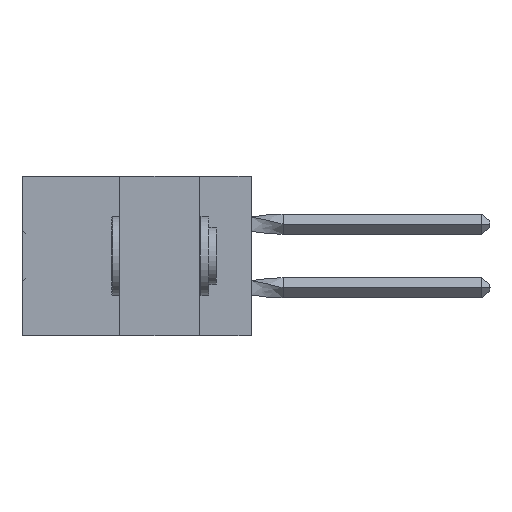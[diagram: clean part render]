
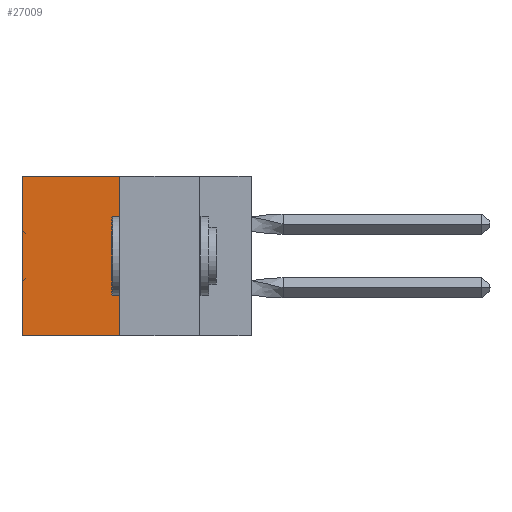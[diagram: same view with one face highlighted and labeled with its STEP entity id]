
A CAD part, left-side view. The second image highlights one B-rep face of the part: STEP entity #27009.
In plain terms, the highlighted planar face has unit normal (-1, 0, 0).
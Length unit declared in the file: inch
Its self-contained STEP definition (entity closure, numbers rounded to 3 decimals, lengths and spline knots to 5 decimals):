
#629 = VECTOR ( 'NONE', #10240, 39.37008 ) ;
#926 = ORIENTED_EDGE ( 'NONE', *, *, #4383, .F. ) ;
#1847 = CARTESIAN_POINT ( 'NONE',  ( 0.305, 0.413, -0.5 ) ) ;
#2015 = ORIENTED_EDGE ( 'NONE', *, *, #31952, .T. ) ;
#3936 = VERTEX_POINT ( 'NONE', #17953 ) ;
#4383 = EDGE_CURVE ( 'NONE', #3936, #9345, #38222, .T. ) ;
#5533 = EDGE_LOOP ( 'NONE', ( #58918, #926, #56568, #2015 ) ) ;
#8923 = VECTOR ( 'NONE', #50853, 39.37008 ) ;
#9345 = VERTEX_POINT ( 'NONE', #12733 ) ;
#10240 = DIRECTION ( 'NONE',  ( 0., 0., -1. ) ) ;
#10301 = LINE ( 'NONE', #25696, #34538 ) ;
#12241 = PLANE ( 'NONE',  #36626 ) ;
#12733 = CARTESIAN_POINT ( 'NONE',  ( 0.305, 0.72, -0.5 ) ) ;
#17953 = CARTESIAN_POINT ( 'NONE',  ( 0.305, 0.413, -0.5 ) ) ;
#19548 = CARTESIAN_POINT ( 'NONE',  ( 0.305, 0.413, -0.5 ) ) ;
#19824 = VERTEX_POINT ( 'NONE', #19971 ) ;
#19971 = CARTESIAN_POINT ( 'NONE',  ( 0.305, 0.413, 0. ) ) ;
#20335 = LINE ( 'NONE', #19548, #629 ) ;
#21225 = EDGE_CURVE ( 'NONE', #19824, #3936, #20335, .T. ) ;
#25521 = CARTESIAN_POINT ( 'NONE',  ( 0.305, 0.413, -0.5 ) ) ;
#25696 = CARTESIAN_POINT ( 'NONE',  ( 0.305, 0.72, -0.5 ) ) ;
#27009 = ADVANCED_FACE ( 'NONE', ( #57143 ), #12241, .F. ) ;
#31952 = EDGE_CURVE ( 'NONE', #19824, #47423, #58804, .T. ) ;
#34538 = VECTOR ( 'NONE', #59500, 39.37008 ) ;
#35964 = CARTESIAN_POINT ( 'NONE',  ( 0.305, 0.72, 0. ) ) ;
#36626 = AXIS2_PLACEMENT_3D ( 'NONE', #1847, #50872, #59964 ) ;
#36931 = CARTESIAN_POINT ( 'NONE',  ( 0.305, 0.413, 0. ) ) ;
#38222 = LINE ( 'NONE', #25521, #57823 ) ;
#47423 = VERTEX_POINT ( 'NONE', #35964 ) ;
#50168 = EDGE_CURVE ( 'NONE', #47423, #9345, #10301, .T. ) ;
#50853 = DIRECTION ( 'NONE',  ( 0., 1., 0. ) ) ;
#50872 = DIRECTION ( 'NONE',  ( 1., 0., 0. ) ) ;
#54659 = DIRECTION ( 'NONE',  ( 0., 1., 0. ) ) ;
#56568 = ORIENTED_EDGE ( 'NONE', *, *, #21225, .F. ) ;
#57143 = FACE_OUTER_BOUND ( 'NONE', #5533, .T. ) ;
#57823 = VECTOR ( 'NONE', #54659, 39.37008 ) ;
#58804 = LINE ( 'NONE', #36931, #8923 ) ;
#58918 = ORIENTED_EDGE ( 'NONE', *, *, #50168, .T. ) ;
#59500 = DIRECTION ( 'NONE',  ( 0., 0., -1. ) ) ;
#59964 = DIRECTION ( 'NONE',  ( 0., 0., -1. ) ) ;
